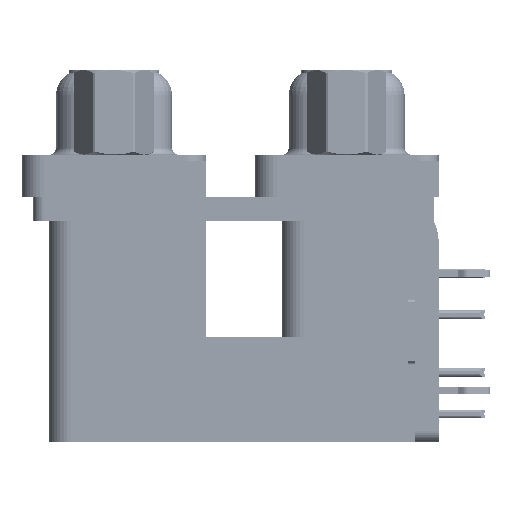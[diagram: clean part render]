
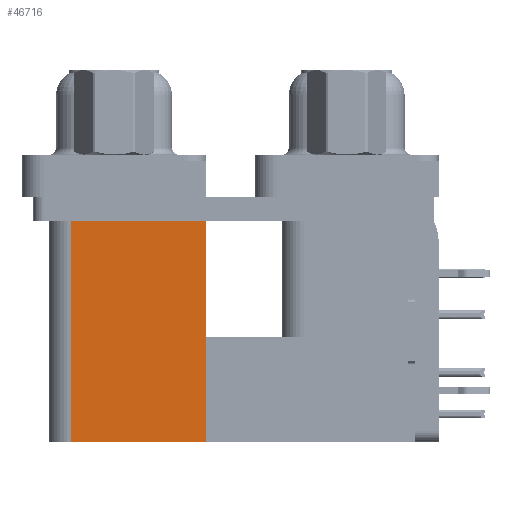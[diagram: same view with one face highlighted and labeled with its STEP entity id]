
A CAD part, left-side view. The second image highlights one B-rep face of the part: STEP entity #46716.
In plain terms, the highlighted planar face has unit normal (-1, 0, 0).
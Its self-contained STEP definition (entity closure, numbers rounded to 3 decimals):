
#2960 = DIRECTION ( 'NONE',  ( 0., 1., 0. ) ) ;
#3184 = EDGE_CURVE ( 'NONE', #27463, #59842, #27417, .T. ) ;
#3936 = FACE_OUTER_BOUND ( 'NONE', #59414, .T. ) ;
#6488 = VECTOR ( 'NONE', #49421, 1000. ) ;
#8114 = LINE ( 'NONE', #45933, #19958 ) ;
#14262 = DIRECTION ( 'NONE',  ( 0., 1., 0. ) ) ;
#19759 = PLANE ( 'NONE',  #35948 ) ;
#19958 = VECTOR ( 'NONE', #2960, 1000. ) ;
#20796 = CARTESIAN_POINT ( 'NONE',  ( 3.7, 9.6, -19.2 ) ) ;
#23957 = DIRECTION ( 'NONE',  ( 0., 1., 0. ) ) ;
#24769 = VECTOR ( 'NONE', #23957, 1000. ) ;
#27092 = VECTOR ( 'NONE', #50263, 1000. ) ;
#27417 = LINE ( 'NONE', #39110, #6488 ) ;
#27463 = VERTEX_POINT ( 'NONE', #30145 ) ;
#27795 = EDGE_CURVE ( 'NONE', #59842, #53629, #56556, .T. ) ;
#30145 = CARTESIAN_POINT ( 'NONE',  ( 3.7, 9.6, -19.2 ) ) ;
#35948 = AXIS2_PLACEMENT_3D ( 'NONE', #20796, #41726, #14262 ) ;
#37486 = CARTESIAN_POINT ( 'NONE',  ( 3.7, 9.6, -2.5 ) ) ;
#39110 = CARTESIAN_POINT ( 'NONE',  ( 3.7, 9.6, -19.2 ) ) ;
#39112 = ORIENTED_EDGE ( 'NONE', *, *, #54863, .F. ) ;
#41726 = DIRECTION ( 'NONE',  ( 1., 0., 0. ) ) ;
#45933 = CARTESIAN_POINT ( 'NONE',  ( 3.7, 9.6, -19.2 ) ) ;
#46379 = ORIENTED_EDGE ( 'NONE', *, *, #3184, .T. ) ;
#46539 = VERTEX_POINT ( 'NONE', #54485 ) ;
#46716 = ADVANCED_FACE ( 'NONE', ( #3936 ), #19759, .F. ) ;
#47747 = ORIENTED_EDGE ( 'NONE', *, *, #64764, .F. ) ;
#48641 = LINE ( 'NONE', #50933, #27092 ) ;
#49421 = DIRECTION ( 'NONE',  ( 0., 0., 1. ) ) ;
#50263 = DIRECTION ( 'NONE',  ( 0., 0., 1. ) ) ;
#50933 = CARTESIAN_POINT ( 'NONE',  ( 3.7, 18.8, -19.2 ) ) ;
#53629 = VERTEX_POINT ( 'NONE', #64218 ) ;
#54485 = CARTESIAN_POINT ( 'NONE',  ( 3.7, 18.8, -19.2 ) ) ;
#54863 = EDGE_CURVE ( 'NONE', #27463, #46539, #8114, .T. ) ;
#56214 = CARTESIAN_POINT ( 'NONE',  ( 3.7, 9.6, -2.5 ) ) ;
#56556 = LINE ( 'NONE', #56214, #24769 ) ;
#59408 = ORIENTED_EDGE ( 'NONE', *, *, #27795, .T. ) ;
#59414 = EDGE_LOOP ( 'NONE', ( #59408, #47747, #39112, #46379 ) ) ;
#59842 = VERTEX_POINT ( 'NONE', #37486 ) ;
#64218 = CARTESIAN_POINT ( 'NONE',  ( 3.7, 18.8, -2.5 ) ) ;
#64764 = EDGE_CURVE ( 'NONE', #46539, #53629, #48641, .T. ) ;
